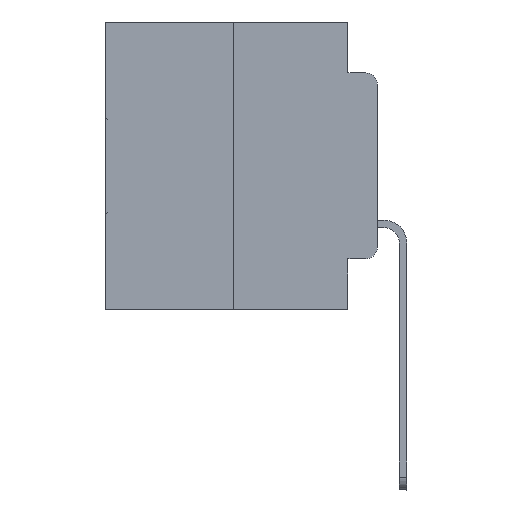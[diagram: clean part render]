
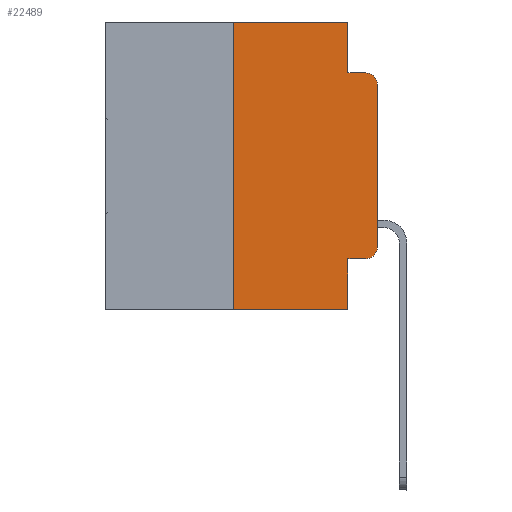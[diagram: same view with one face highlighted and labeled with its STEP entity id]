
A CAD part, left-side view. The second image highlights one B-rep face of the part: STEP entity #22489.
In plain terms, the highlighted planar face has unit normal (-1, 0, 0).
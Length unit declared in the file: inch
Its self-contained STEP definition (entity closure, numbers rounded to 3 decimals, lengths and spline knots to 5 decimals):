
#767 = VERTEX_POINT ( 'NONE', #2724 ) ;
#902 = DIRECTION ( 'NONE',  ( -1., 0., 0. ) ) ;
#922 = LINE ( 'NONE', #22729, #18509 ) ;
#1342 = CARTESIAN_POINT ( 'NONE',  ( 0., 0.02, -0.4115 ) ) ;
#1832 = CARTESIAN_POINT ( 'NONE',  ( 0., 0.051, 0. ) ) ;
#2196 = VERTEX_POINT ( 'NONE', #2226 ) ;
#2226 = CARTESIAN_POINT ( 'NONE',  ( 0., 0.051, -0.4115 ) ) ;
#2386 = EDGE_CURVE ( 'NONE', #3901, #25358, #922, .T. ) ;
#2470 = DIRECTION ( 'NONE',  ( 0., 0., -1. ) ) ;
#2724 = CARTESIAN_POINT ( 'NONE',  ( 0., 0.051, -0.0885 ) ) ;
#2803 = LINE ( 'NONE', #17424, #25159 ) ;
#3666 = VERTEX_POINT ( 'NONE', #20118 ) ;
#3901 = VERTEX_POINT ( 'NONE', #9006 ) ;
#4356 = VECTOR ( 'NONE', #24467, 39.37008 ) ;
#4490 = EDGE_CURVE ( 'NONE', #7117, #3666, #5561, .T. ) ;
#4866 = EDGE_CURVE ( 'NONE', #767, #23627, #25377, .T. ) ;
#4934 = ORIENTED_EDGE ( 'NONE', *, *, #12044, .T. ) ;
#5561 = LINE ( 'NONE', #7499, #5726 ) ;
#5600 = EDGE_LOOP ( 'NONE', ( #18805, #31878, #15521, #6807, #5701, #16695, #25367, #29915, #19120, #4934 ) ) ;
#5701 = ORIENTED_EDGE ( 'NONE', *, *, #6233, .F. ) ;
#5726 = VECTOR ( 'NONE', #8152, 39.37008 ) ;
#6233 = EDGE_CURVE ( 'NONE', #10174, #8252, #31047, .T. ) ;
#6807 = ORIENTED_EDGE ( 'NONE', *, *, #26378, .F. ) ;
#7117 = VERTEX_POINT ( 'NONE', #31413 ) ;
#7328 = LINE ( 'NONE', #17586, #25099 ) ;
#7462 = DIRECTION ( 'NONE',  ( 0., -1., 0. ) ) ;
#7499 = CARTESIAN_POINT ( 'NONE',  ( 0., 0.473, -0.5 ) ) ;
#7626 = AXIS2_PLACEMENT_3D ( 'NONE', #30428, #20951, #18009 ) ;
#8152 = DIRECTION ( 'NONE',  ( 0., -1., 0. ) ) ;
#8252 = VERTEX_POINT ( 'NONE', #31102 ) ;
#8866 = DIRECTION ( 'NONE',  ( 0., -1., 0. ) ) ;
#8945 = VECTOR ( 'NONE', #8866, 39.37008 ) ;
#9006 = CARTESIAN_POINT ( 'NONE',  ( 0., 0., -0.3915 ) ) ;
#9127 = LINE ( 'NONE', #1832, #17872 ) ;
#9528 = EDGE_CURVE ( 'NONE', #2196, #13707, #16640, .T. ) ;
#9917 = CARTESIAN_POINT ( 'NONE',  ( 0., 0.051, -0.0885 ) ) ;
#10174 = VERTEX_POINT ( 'NONE', #20028 ) ;
#10274 = DIRECTION ( 'NONE',  ( 0., 0., 1. ) ) ;
#10451 = VECTOR ( 'NONE', #7462, 39.37008 ) ;
#11390 = PLANE ( 'NONE',  #27646 ) ;
#12044 = EDGE_CURVE ( 'NONE', #13707, #3901, #31569, .T. ) ;
#13707 = VERTEX_POINT ( 'NONE', #1342 ) ;
#13962 = CIRCLE ( 'NONE', #23869, 0.02 ) ;
#15521 = ORIENTED_EDGE ( 'NONE', *, *, #4866, .F. ) ;
#15826 = DIRECTION ( 'NONE',  ( 0., 0., -1. ) ) ;
#16640 = LINE ( 'NONE', #23979, #4356 ) ;
#16695 = ORIENTED_EDGE ( 'NONE', *, *, #27666, .F. ) ;
#17424 = CARTESIAN_POINT ( 'NONE',  ( 0., 0.25, 0. ) ) ;
#17586 = CARTESIAN_POINT ( 'NONE',  ( 0., 0.051, 0. ) ) ;
#17872 = VECTOR ( 'NONE', #24275, 39.37008 ) ;
#18009 = DIRECTION ( 'NONE',  ( 0., 0., -1. ) ) ;
#18509 = VECTOR ( 'NONE', #30386, 39.37008 ) ;
#18805 = ORIENTED_EDGE ( 'NONE', *, *, #2386, .T. ) ;
#19120 = ORIENTED_EDGE ( 'NONE', *, *, #9528, .T. ) ;
#20028 = CARTESIAN_POINT ( 'NONE',  ( 0., 0.25, 0. ) ) ;
#20118 = CARTESIAN_POINT ( 'NONE',  ( 0., 0.051, -0.5 ) ) ;
#20137 = EDGE_CURVE ( 'NONE', #25358, #23627, #13962, .T. ) ;
#20253 = CARTESIAN_POINT ( 'NONE',  ( 0., 0.02, -0.0885 ) ) ;
#20951 = DIRECTION ( 'NONE',  ( -1., 0., 0. ) ) ;
#21323 = FACE_OUTER_BOUND ( 'NONE', #5600, .T. ) ;
#22489 = ADVANCED_FACE ( 'NONE', ( #21323 ), #11390, .F. ) ;
#22729 = CARTESIAN_POINT ( 'NONE',  ( 0., 0., 0. ) ) ;
#23627 = VERTEX_POINT ( 'NONE', #20253 ) ;
#23869 = AXIS2_PLACEMENT_3D ( 'NONE', #25615, #902, #15826 ) ;
#23979 = CARTESIAN_POINT ( 'NONE',  ( 0., 0.051, -0.4115 ) ) ;
#24275 = DIRECTION ( 'NONE',  ( 0., 0., -1. ) ) ;
#24467 = DIRECTION ( 'NONE',  ( 0., -1., 0. ) ) ;
#25099 = VECTOR ( 'NONE', #2470, 39.37008 ) ;
#25159 = VECTOR ( 'NONE', #10274, 39.37008 ) ;
#25358 = VERTEX_POINT ( 'NONE', #31978 ) ;
#25367 = ORIENTED_EDGE ( 'NONE', *, *, #4490, .T. ) ;
#25377 = LINE ( 'NONE', #9917, #10451 ) ;
#25615 = CARTESIAN_POINT ( 'NONE',  ( 0., 0.02, -0.1085 ) ) ;
#26378 = EDGE_CURVE ( 'NONE', #8252, #767, #7328, .T. ) ;
#26544 = DIRECTION ( 'NONE',  ( 1., 0., 0. ) ) ;
#27538 = EDGE_CURVE ( 'NONE', #2196, #3666, #9127, .T. ) ;
#27646 = AXIS2_PLACEMENT_3D ( 'NONE', #28356, #26544, #30964 ) ;
#27666 = EDGE_CURVE ( 'NONE', #7117, #10174, #2803, .T. ) ;
#28356 = CARTESIAN_POINT ( 'NONE',  ( 0., 0.473, 0. ) ) ;
#29915 = ORIENTED_EDGE ( 'NONE', *, *, #27538, .F. ) ;
#30386 = DIRECTION ( 'NONE',  ( 0., 0., 1. ) ) ;
#30428 = CARTESIAN_POINT ( 'NONE',  ( 0., 0.02, -0.3915 ) ) ;
#30964 = DIRECTION ( 'NONE',  ( 0., 0., -1. ) ) ;
#31047 = LINE ( 'NONE', #31215, #8945 ) ;
#31102 = CARTESIAN_POINT ( 'NONE',  ( 0., 0.051, 0. ) ) ;
#31215 = CARTESIAN_POINT ( 'NONE',  ( 0., 0.473, 0. ) ) ;
#31413 = CARTESIAN_POINT ( 'NONE',  ( 0., 0.25, -0.5 ) ) ;
#31569 = CIRCLE ( 'NONE', #7626, 0.02 ) ;
#31878 = ORIENTED_EDGE ( 'NONE', *, *, #20137, .T. ) ;
#31978 = CARTESIAN_POINT ( 'NONE',  ( 0., 0., -0.1085 ) ) ;
